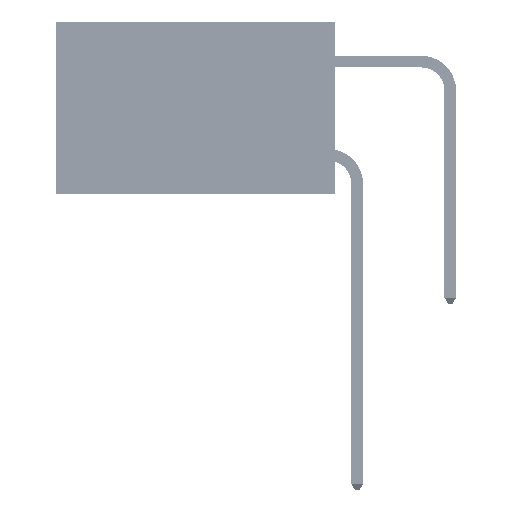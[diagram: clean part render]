
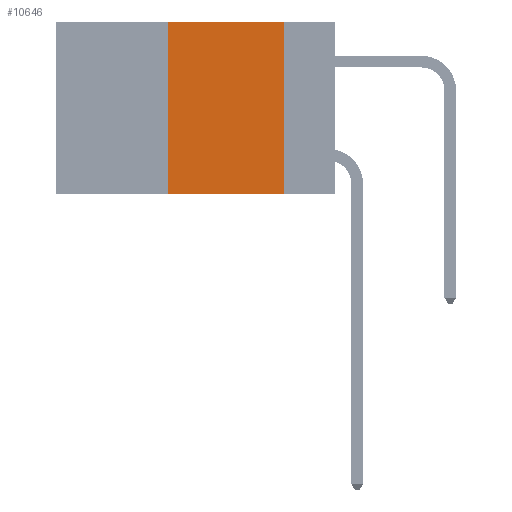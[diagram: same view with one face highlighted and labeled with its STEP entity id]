
A CAD part, left-side view. The second image highlights one B-rep face of the part: STEP entity #10646.
In plain terms, the highlighted planar face has unit normal (-1, 0, 0).
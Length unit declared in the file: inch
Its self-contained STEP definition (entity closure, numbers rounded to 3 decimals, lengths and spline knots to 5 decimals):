
#3113 = CARTESIAN_POINT ( 'NONE',  ( 0., 0.11, 0. ) ) ;
#4275 = CARTESIAN_POINT ( 'NONE',  ( 0., 0.6, -0.37 ) ) ;
#8418 = CARTESIAN_POINT ( 'NONE',  ( 0., 0.6, 0. ) ) ;
#8949 = CARTESIAN_POINT ( 'NONE',  ( 0., 0.6, 0. ) ) ;
#9854 = DIRECTION ( 'NONE',  ( 0., 0., 1. ) ) ;
#10646 = ADVANCED_FACE ( 'NONE', ( #44422 ), #29925, .F. ) ;
#11092 = AXIS2_PLACEMENT_3D ( 'NONE', #8949, #12618, #38008 ) ;
#12618 = DIRECTION ( 'NONE',  ( 1., 0., 0. ) ) ;
#12900 = LINE ( 'NONE', #4275, #32223 ) ;
#16177 = VERTEX_POINT ( 'NONE', #18113 ) ;
#16391 = VECTOR ( 'NONE', #33862, 39.37008 ) ;
#18113 = CARTESIAN_POINT ( 'NONE',  ( 0., 0.11, -0.37 ) ) ;
#18796 = DIRECTION ( 'NONE',  ( 0., -1., 0. ) ) ;
#18852 = ORIENTED_EDGE ( 'NONE', *, *, #40013, .F. ) ;
#18919 = EDGE_CURVE ( 'NONE', #34769, #16177, #12900, .T. ) ;
#20114 = ORIENTED_EDGE ( 'NONE', *, *, #35010, .F. ) ;
#20721 = CARTESIAN_POINT ( 'NONE',  ( 0., 0.36, 0. ) ) ;
#25304 = VECTOR ( 'NONE', #32174, 39.37008 ) ;
#27238 = ORIENTED_EDGE ( 'NONE', *, *, #38338, .F. ) ;
#28518 = ORIENTED_EDGE ( 'NONE', *, *, #18919, .T. ) ;
#29925 = PLANE ( 'NONE',  #11092 ) ;
#30616 = CARTESIAN_POINT ( 'NONE',  ( 0., 0.36, -0.37 ) ) ;
#31807 = VECTOR ( 'NONE', #9854, 39.37008 ) ;
#32174 = DIRECTION ( 'NONE',  ( 0., 0., -1. ) ) ;
#32223 = VECTOR ( 'NONE', #18796, 39.37008 ) ;
#33862 = DIRECTION ( 'NONE',  ( 0., -1., 0. ) ) ;
#34769 = VERTEX_POINT ( 'NONE', #30616 ) ;
#34963 = CARTESIAN_POINT ( 'NONE',  ( 0., 0.36, 0. ) ) ;
#35010 = EDGE_CURVE ( 'NONE', #45431, #16177, #43474, .T. ) ;
#35234 = LINE ( 'NONE', #20721, #31807 ) ;
#35539 = CARTESIAN_POINT ( 'NONE',  ( 0., 0.11, 0. ) ) ;
#35695 = LINE ( 'NONE', #8418, #16391 ) ;
#38008 = DIRECTION ( 'NONE',  ( 0., 0., -1. ) ) ;
#38338 = EDGE_CURVE ( 'NONE', #34769, #44625, #35234, .T. ) ;
#39494 = EDGE_LOOP ( 'NONE', ( #20114, #18852, #27238, #28518 ) ) ;
#40013 = EDGE_CURVE ( 'NONE', #44625, #45431, #35695, .T. ) ;
#43474 = LINE ( 'NONE', #3113, #25304 ) ;
#44422 = FACE_OUTER_BOUND ( 'NONE', #39494, .T. ) ;
#44625 = VERTEX_POINT ( 'NONE', #34963 ) ;
#45431 = VERTEX_POINT ( 'NONE', #35539 ) ;
